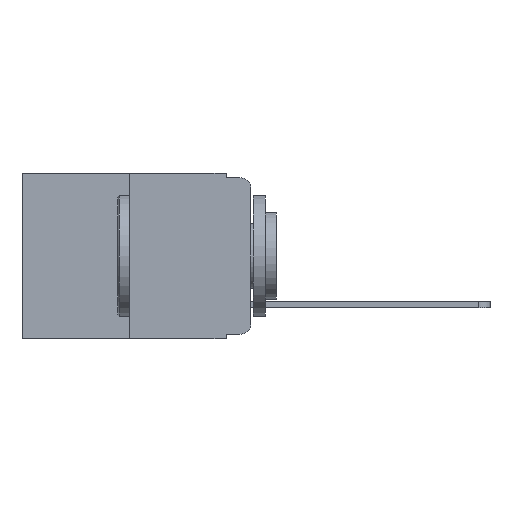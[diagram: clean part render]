
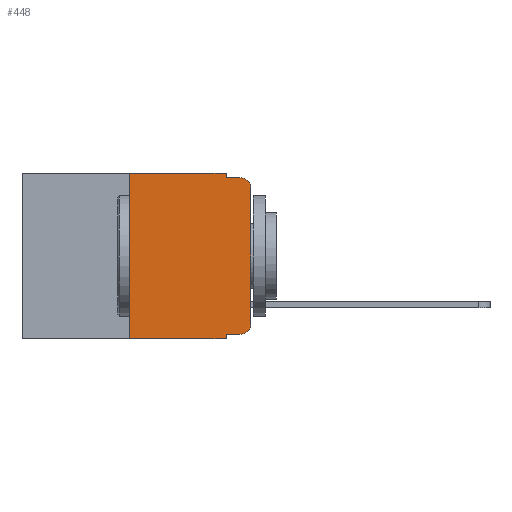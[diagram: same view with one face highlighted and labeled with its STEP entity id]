
A CAD part, left-side view. The second image highlights one B-rep face of the part: STEP entity #448.
In plain terms, the highlighted planar face has unit normal (-1, 0, 0).
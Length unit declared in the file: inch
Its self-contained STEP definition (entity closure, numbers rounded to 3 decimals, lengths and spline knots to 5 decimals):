
#218 = VERTEX_POINT ( 'NONE', #20606 ) ;
#448 = ADVANCED_FACE ( 'NONE', ( #9199 ), #9658, .F. ) ;
#602 = ORIENTED_EDGE ( 'NONE', *, *, #8471, .F. ) ;
#711 = EDGE_CURVE ( 'NONE', #18844, #20816, #21457, .T. ) ;
#1282 = CARTESIAN_POINT ( 'NONE',  ( 0., 0.051, 0. ) ) ;
#1355 = EDGE_CURVE ( 'NONE', #23664, #9906, #15617, .T. ) ;
#1739 = CARTESIAN_POINT ( 'NONE',  ( 0., 0.051, -0.01 ) ) ;
#2294 = VECTOR ( 'NONE', #3932, 39.37008 ) ;
#3932 = DIRECTION ( 'NONE',  ( 0., -1., 0. ) ) ;
#4544 = DIRECTION ( 'NONE',  ( 0., 0., -1. ) ) ;
#4955 = CARTESIAN_POINT ( 'NONE',  ( 0., 0.051, -0.333 ) ) ;
#5023 = DIRECTION ( 'NONE',  ( 0., 0., -1. ) ) ;
#5344 = DIRECTION ( 'NONE',  ( 0., 0., 1. ) ) ;
#6473 = LINE ( 'NONE', #22041, #7431 ) ;
#7256 = EDGE_LOOP ( 'NONE', ( #10171, #8377, #8891, #9758, #24756, #20434, #25954, #602, #9762, #26519 ) ) ;
#7431 = VECTOR ( 'NONE', #5344, 39.37008 ) ;
#8058 = CARTESIAN_POINT ( 'NONE',  ( 0., 0.02, -0.01 ) ) ;
#8100 = AXIS2_PLACEMENT_3D ( 'NONE', #12232, #26689, #4544 ) ;
#8113 = EDGE_CURVE ( 'NONE', #20816, #11024, #13422, .T. ) ;
#8377 = ORIENTED_EDGE ( 'NONE', *, *, #10598, .T. ) ;
#8396 = DIRECTION ( 'NONE',  ( 0., 0., -1. ) ) ;
#8471 = EDGE_CURVE ( 'NONE', #22979, #218, #23434, .T. ) ;
#8891 = ORIENTED_EDGE ( 'NONE', *, *, #8113, .F. ) ;
#9199 = FACE_OUTER_BOUND ( 'NONE', #7256, .T. ) ;
#9365 = EDGE_CURVE ( 'NONE', #13263, #18844, #17552, .T. ) ;
#9658 = PLANE ( 'NONE',  #19675 ) ;
#9758 = ORIENTED_EDGE ( 'NONE', *, *, #711, .F. ) ;
#9762 = ORIENTED_EDGE ( 'NONE', *, *, #22350, .T. ) ;
#9906 = VERTEX_POINT ( 'NONE', #24422 ) ;
#10036 = DIRECTION ( 'NONE',  ( 0., 0., 1. ) ) ;
#10171 = ORIENTED_EDGE ( 'NONE', *, *, #1355, .T. ) ;
#10392 = CIRCLE ( 'NONE', #8100, 0.02 ) ;
#10463 = DIRECTION ( 'NONE',  ( -1., 0., 0. ) ) ;
#10496 = VECTOR ( 'NONE', #23585, 39.37008 ) ;
#10598 = EDGE_CURVE ( 'NONE', #9906, #11024, #10392, .T. ) ;
#11024 = VERTEX_POINT ( 'NONE', #8058 ) ;
#11419 = VECTOR ( 'NONE', #10036, 39.37008 ) ;
#11884 = CARTESIAN_POINT ( 'NONE',  ( 0., 0., 0. ) ) ;
#12232 = CARTESIAN_POINT ( 'NONE',  ( 0., 0.02, -0.03 ) ) ;
#12396 = CARTESIAN_POINT ( 'NONE',  ( 0., 0.25, 0. ) ) ;
#12624 = CARTESIAN_POINT ( 'NONE',  ( 0., 0.051, 0. ) ) ;
#13263 = VERTEX_POINT ( 'NONE', #12396 ) ;
#13422 = LINE ( 'NONE', #1739, #25077 ) ;
#13438 = AXIS2_PLACEMENT_3D ( 'NONE', #20942, #10463, #8396 ) ;
#13506 = DIRECTION ( 'NONE',  ( 1., 0., 0. ) ) ;
#14174 = CARTESIAN_POINT ( 'NONE',  ( 0., 0.02, -0.333 ) ) ;
#15199 = CIRCLE ( 'NONE', #13438, 0.02 ) ;
#15211 = CARTESIAN_POINT ( 'NONE',  ( 0., 0.051, -0.333 ) ) ;
#15327 = VECTOR ( 'NONE', #5023, 39.37008 ) ;
#15617 = LINE ( 'NONE', #11884, #11419 ) ;
#15679 = VERTEX_POINT ( 'NONE', #14174 ) ;
#16895 = VECTOR ( 'NONE', #21166, 39.37008 ) ;
#17012 = VECTOR ( 'NONE', #21647, 39.37008 ) ;
#17552 = LINE ( 'NONE', #25167, #16895 ) ;
#18761 = EDGE_CURVE ( 'NONE', #15679, #23664, #15199, .T. ) ;
#18844 = VERTEX_POINT ( 'NONE', #12624 ) ;
#19675 = AXIS2_PLACEMENT_3D ( 'NONE', #24152, #13506, #23627 ) ;
#19828 = EDGE_CURVE ( 'NONE', #21573, #218, #24276, .T. ) ;
#20352 = EDGE_CURVE ( 'NONE', #21573, #13263, #6473, .T. ) ;
#20434 = ORIENTED_EDGE ( 'NONE', *, *, #20352, .F. ) ;
#20606 = CARTESIAN_POINT ( 'NONE',  ( 0., 0.051, -0.343 ) ) ;
#20816 = VERTEX_POINT ( 'NONE', #22281 ) ;
#20942 = CARTESIAN_POINT ( 'NONE',  ( 0., 0.02, -0.313 ) ) ;
#21166 = DIRECTION ( 'NONE',  ( 0., -1., 0. ) ) ;
#21199 = LINE ( 'NONE', #4955, #17012 ) ;
#21457 = LINE ( 'NONE', #21623, #15327 ) ;
#21573 = VERTEX_POINT ( 'NONE', #25309 ) ;
#21623 = CARTESIAN_POINT ( 'NONE',  ( 0., 0.051, 0. ) ) ;
#21647 = DIRECTION ( 'NONE',  ( 0., -1., 0. ) ) ;
#22041 = CARTESIAN_POINT ( 'NONE',  ( 0., 0.25, 0. ) ) ;
#22281 = CARTESIAN_POINT ( 'NONE',  ( 0., 0.051, -0.01 ) ) ;
#22350 = EDGE_CURVE ( 'NONE', #22979, #15679, #21199, .T. ) ;
#22869 = CARTESIAN_POINT ( 'NONE',  ( 0., 0.473, -0.343 ) ) ;
#22979 = VERTEX_POINT ( 'NONE', #15211 ) ;
#23434 = LINE ( 'NONE', #1282, #10496 ) ;
#23585 = DIRECTION ( 'NONE',  ( 0., 0., -1. ) ) ;
#23593 = CARTESIAN_POINT ( 'NONE',  ( 0., 0., -0.313 ) ) ;
#23627 = DIRECTION ( 'NONE',  ( 0., 0., -1. ) ) ;
#23664 = VERTEX_POINT ( 'NONE', #23593 ) ;
#24152 = CARTESIAN_POINT ( 'NONE',  ( 0., 0.473, 0. ) ) ;
#24276 = LINE ( 'NONE', #22869, #2294 ) ;
#24422 = CARTESIAN_POINT ( 'NONE',  ( 0., 0., -0.03 ) ) ;
#24756 = ORIENTED_EDGE ( 'NONE', *, *, #9365, .F. ) ;
#25077 = VECTOR ( 'NONE', #26575, 39.37008 ) ;
#25167 = CARTESIAN_POINT ( 'NONE',  ( 0., 0.473, 0. ) ) ;
#25309 = CARTESIAN_POINT ( 'NONE',  ( 0., 0.25, -0.343 ) ) ;
#25954 = ORIENTED_EDGE ( 'NONE', *, *, #19828, .T. ) ;
#26519 = ORIENTED_EDGE ( 'NONE', *, *, #18761, .T. ) ;
#26575 = DIRECTION ( 'NONE',  ( 0., -1., 0. ) ) ;
#26689 = DIRECTION ( 'NONE',  ( -1., 0., 0. ) ) ;
